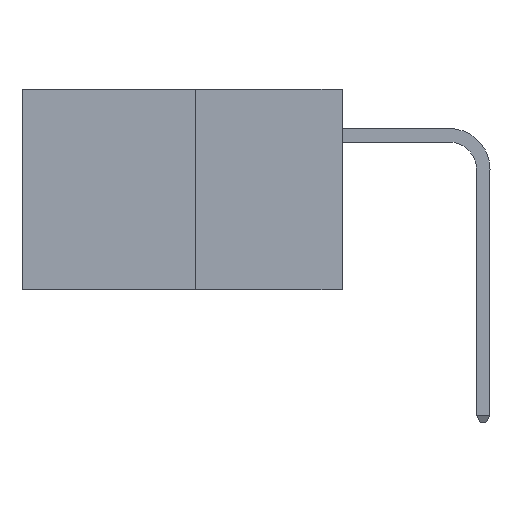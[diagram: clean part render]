
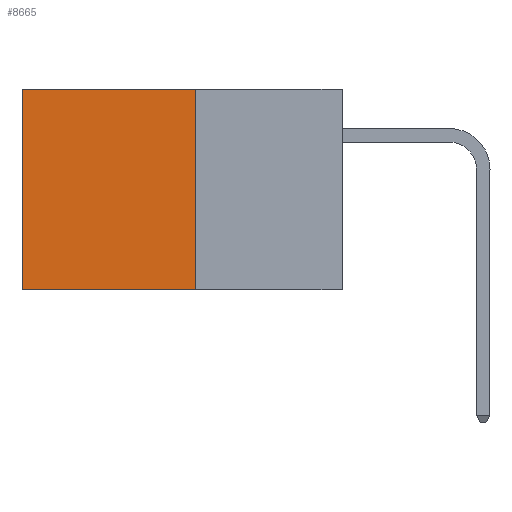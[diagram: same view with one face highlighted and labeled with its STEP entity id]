
A CAD part, left-side view. The second image highlights one B-rep face of the part: STEP entity #8665.
In plain terms, the highlighted planar face has unit normal (-1, 0, 0).
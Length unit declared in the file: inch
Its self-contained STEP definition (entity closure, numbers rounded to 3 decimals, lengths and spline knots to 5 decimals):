
#59 = LINE ( 'NONE', #10978, #11188 ) ;
#135 = ORIENTED_EDGE ( 'NONE', *, *, #12143, .T. ) ;
#142 = EDGE_CURVE ( 'NONE', #5412, #5104, #12596, .T. ) ;
#206 = ORIENTED_EDGE ( 'NONE', *, *, #6038, .F. ) ;
#239 = ORIENTED_EDGE ( 'NONE', *, *, #142, .F. ) ;
#271 = ORIENTED_EDGE ( 'NONE', *, *, #2274, .T. ) ;
#2243 = DIRECTION ( 'NONE',  ( 0., 0., -1. ) ) ;
#2274 = EDGE_CURVE ( 'NONE', #5412, #6609, #3934, .T. ) ;
#2442 = CARTESIAN_POINT ( 'NONE',  ( 0.277, 0.59, 0. ) ) ;
#3081 = VECTOR ( 'NONE', #10000, 39.37008 ) ;
#3124 = DIRECTION ( 'NONE',  ( 0., 0., -1. ) ) ;
#3310 = CARTESIAN_POINT ( 'NONE',  ( 0.277, 0.27, -0.37 ) ) ;
#3736 = LINE ( 'NONE', #13145, #3081 ) ;
#3835 = FACE_OUTER_BOUND ( 'NONE', #4587, .T. ) ;
#3934 = LINE ( 'NONE', #7214, #9446 ) ;
#4320 = VERTEX_POINT ( 'NONE', #9540 ) ;
#4587 = EDGE_LOOP ( 'NONE', ( #135, #206, #239, #271 ) ) ;
#5104 = VERTEX_POINT ( 'NONE', #8667 ) ;
#5354 = CARTESIAN_POINT ( 'NONE',  ( 0.277, 0.27, -0.37 ) ) ;
#5412 = VERTEX_POINT ( 'NONE', #7892 ) ;
#6038 = EDGE_CURVE ( 'NONE', #5104, #4320, #59, .T. ) ;
#6609 = VERTEX_POINT ( 'NONE', #2442 ) ;
#7214 = CARTESIAN_POINT ( 'NONE',  ( 0.277, 0.27, 0. ) ) ;
#7493 = PLANE ( 'NONE',  #8195 ) ;
#7874 = DIRECTION ( 'NONE',  ( 0., 1., 0. ) ) ;
#7892 = CARTESIAN_POINT ( 'NONE',  ( 0.277, 0.27, 0. ) ) ;
#8195 = AXIS2_PLACEMENT_3D ( 'NONE', #3310, #8538, #2243 ) ;
#8538 = DIRECTION ( 'NONE',  ( 1., 0., 0. ) ) ;
#8665 = ADVANCED_FACE ( 'NONE', ( #3835 ), #7493, .F. ) ;
#8667 = CARTESIAN_POINT ( 'NONE',  ( 0.277, 0.27, -0.37 ) ) ;
#9446 = VECTOR ( 'NONE', #12055, 39.37008 ) ;
#9540 = CARTESIAN_POINT ( 'NONE',  ( 0.277, 0.59, -0.37 ) ) ;
#9789 = VECTOR ( 'NONE', #3124, 39.37008 ) ;
#10000 = DIRECTION ( 'NONE',  ( 0., 0., -1. ) ) ;
#10978 = CARTESIAN_POINT ( 'NONE',  ( 0.277, 0.27, -0.37 ) ) ;
#11188 = VECTOR ( 'NONE', #7874, 39.37008 ) ;
#12055 = DIRECTION ( 'NONE',  ( 0., 1., 0. ) ) ;
#12143 = EDGE_CURVE ( 'NONE', #6609, #4320, #3736, .T. ) ;
#12596 = LINE ( 'NONE', #5354, #9789 ) ;
#13145 = CARTESIAN_POINT ( 'NONE',  ( 0.277, 0.59, -0.37 ) ) ;
